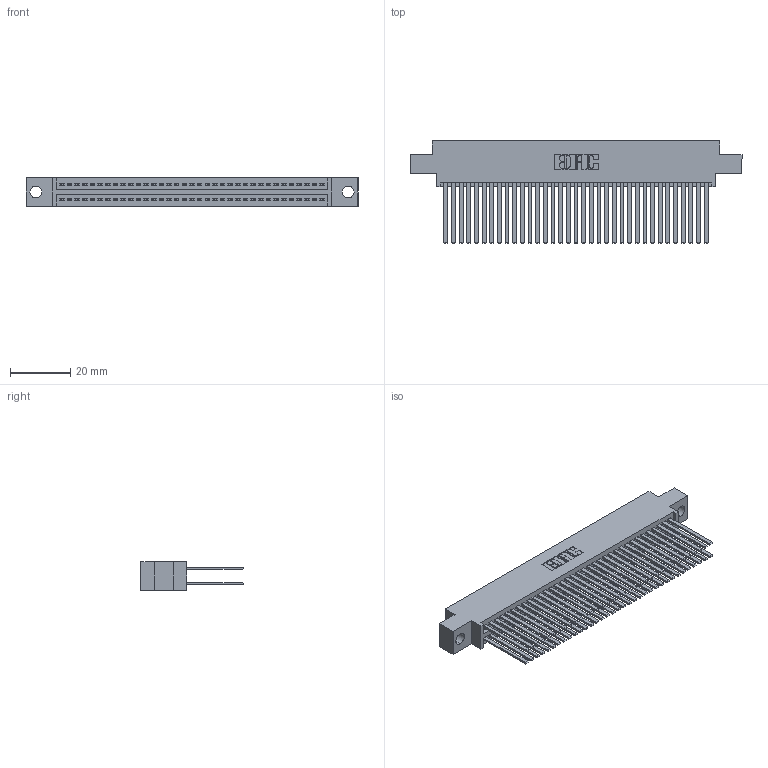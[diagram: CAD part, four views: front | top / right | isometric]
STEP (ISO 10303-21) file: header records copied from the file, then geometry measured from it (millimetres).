
FILE_DESCRIPTION (( 'STEP AP203' ), '1' );
FILE_NAME ('345-070-544-804.STEP', '2021-05-20T08:25:48', ( '' ), ( '' ), 'SwSTEP 2.0', 'SolidWorks 2020', '' );
FILE_SCHEMA (( 'CONFIG_CONTROL_DESIGN' ));
Length unit declared in the file: inch
Products named in the file (3): 345 Part_0.170 Offset - 0.156 Dia-TI; 345-070-544-804; 345-292-001_345-293-144
Assembly tree (71 placements, depth 2):
  345-070-544-804
    345 Part_0.170 Offset - 0.156 Dia-TI
    345-292-001_345-293-144  x70
Bounding box: 110.11 x 33.96 x 9.4 mm (x, y, z)
Volume: 11393.1 mm3; surface area: 19576.4 mm2
Topology: 71 solids, 71 shells, 3224 faces, 9559 edges, 6278 vertices
Faces by surface type: plane 2128, cylinder 1096
Entity records: 28771 total; most frequent: CARTESIAN_POINT 4834, ORIENTED_EDGE 4766, DIRECTION 4267, EDGE_CURVE 2383, VECTOR 2115, LINE 2115, VERTEX_POINT 1586, AXIS2_PLACEMENT_3D 1076
